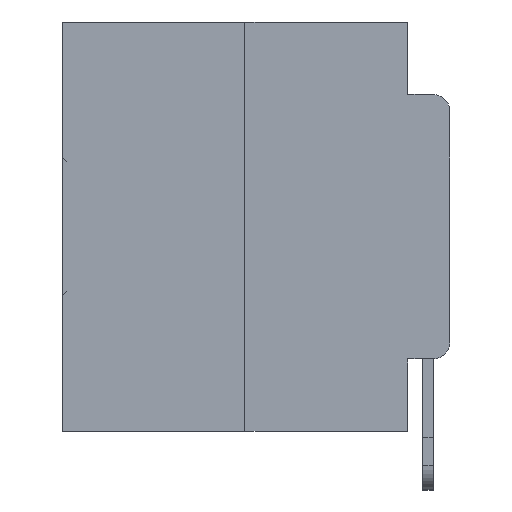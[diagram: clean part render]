
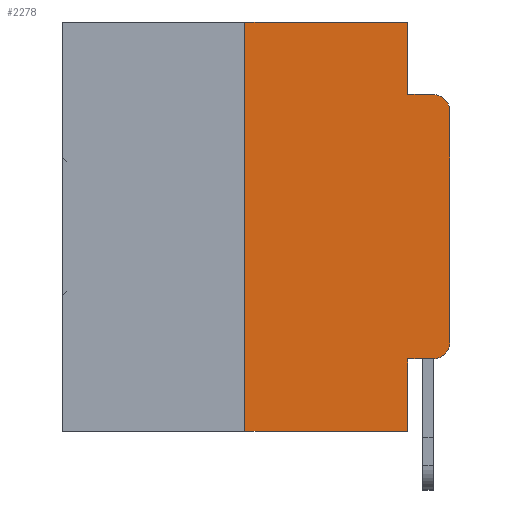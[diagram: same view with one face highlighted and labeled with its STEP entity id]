
A CAD part, left-side view. The second image highlights one B-rep face of the part: STEP entity #2278.
In plain terms, the highlighted planar face has unit normal (-1, 0, 0).
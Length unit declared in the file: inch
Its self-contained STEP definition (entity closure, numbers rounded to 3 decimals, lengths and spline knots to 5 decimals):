
#364 = EDGE_CURVE ( 'NONE', #15188, #6510, #6647, .T. ) ;
#1697 = VERTEX_POINT ( 'NONE', #27695 ) ;
#1783 = ORIENTED_EDGE ( 'NONE', *, *, #17709, .T. ) ;
#1814 = ORIENTED_EDGE ( 'NONE', *, *, #17591, .T. ) ;
#2278 = ADVANCED_FACE ( 'NONE', ( #27817 ), #11247, .F. ) ;
#2886 = EDGE_LOOP ( 'NONE', ( #29940, #19424, #7534, #15975, #30333, #12419, #1783, #5867, #1814, #16765 ) ) ;
#3053 = CIRCLE ( 'NONE', #8954, 0.02 ) ;
#3442 = VECTOR ( 'NONE', #27113, 39.37008 ) ;
#3641 = VERTEX_POINT ( 'NONE', #31999 ) ;
#3981 = EDGE_CURVE ( 'NONE', #6510, #9661, #31100, .T. ) ;
#4026 = EDGE_CURVE ( 'NONE', #1697, #14434, #3053, .T. ) ;
#4853 = DIRECTION ( 'NONE',  ( -1., 0., 0. ) ) ;
#4941 = CARTESIAN_POINT ( 'NONE',  ( 0., 0., -0.3915 ) ) ;
#5048 = CARTESIAN_POINT ( 'NONE',  ( 0., 0.473, -0.5 ) ) ;
#5867 = ORIENTED_EDGE ( 'NONE', *, *, #24782, .F. ) ;
#5984 = VECTOR ( 'NONE', #32079, 39.37008 ) ;
#6510 = VERTEX_POINT ( 'NONE', #27683 ) ;
#6591 = CARTESIAN_POINT ( 'NONE',  ( 0., 0.051, -0.5 ) ) ;
#6647 = LINE ( 'NONE', #26902, #32130 ) ;
#7245 = DIRECTION ( 'NONE',  ( 0., -1., 0. ) ) ;
#7264 = DIRECTION ( 'NONE',  ( 0., 0., -1. ) ) ;
#7534 = ORIENTED_EDGE ( 'NONE', *, *, #21222, .F. ) ;
#7689 = DIRECTION ( 'NONE',  ( 0., -1., 0. ) ) ;
#8711 = DIRECTION ( 'NONE',  ( -1., 0., 0. ) ) ;
#8758 = DIRECTION ( 'NONE',  ( 1., 0., 0. ) ) ;
#8954 = AXIS2_PLACEMENT_3D ( 'NONE', #20085, #4853, #22488 ) ;
#9661 = VERTEX_POINT ( 'NONE', #22463 ) ;
#9944 = DIRECTION ( 'NONE',  ( 0., -1., 0. ) ) ;
#10630 = AXIS2_PLACEMENT_3D ( 'NONE', #21287, #8758, #26061 ) ;
#10743 = CARTESIAN_POINT ( 'NONE',  ( 0., 0.051, -0.0885 ) ) ;
#11247 = PLANE ( 'NONE',  #10630 ) ;
#12419 = ORIENTED_EDGE ( 'NONE', *, *, #28015, .F. ) ;
#12770 = VERTEX_POINT ( 'NONE', #30619 ) ;
#12849 = VECTOR ( 'NONE', #7245, 39.37008 ) ;
#14434 = VERTEX_POINT ( 'NONE', #4941 ) ;
#15188 = VERTEX_POINT ( 'NONE', #20180 ) ;
#15628 = VECTOR ( 'NONE', #7689, 39.37008 ) ;
#15975 = ORIENTED_EDGE ( 'NONE', *, *, #3981, .F. ) ;
#16373 = LINE ( 'NONE', #5048, #15628 ) ;
#16599 = EDGE_CURVE ( 'NONE', #14434, #23954, #25861, .T. ) ;
#16765 = ORIENTED_EDGE ( 'NONE', *, *, #4026, .T. ) ;
#17411 = CARTESIAN_POINT ( 'NONE',  ( 0., 0.051, -0.4115 ) ) ;
#17591 = EDGE_CURVE ( 'NONE', #3641, #1697, #25799, .T. ) ;
#17679 = CARTESIAN_POINT ( 'NONE',  ( 0., 0., 0. ) ) ;
#17709 = EDGE_CURVE ( 'NONE', #12770, #20776, #16373, .T. ) ;
#19424 = ORIENTED_EDGE ( 'NONE', *, *, #26911, .T. ) ;
#20085 = CARTESIAN_POINT ( 'NONE',  ( 0., 0.02, -0.3915 ) ) ;
#20180 = CARTESIAN_POINT ( 'NONE',  ( 0., 0.25, 0. ) ) ;
#20213 = DIRECTION ( 'NONE',  ( 0., 0., -1. ) ) ;
#20776 = VERTEX_POINT ( 'NONE', #6591 ) ;
#21158 = CIRCLE ( 'NONE', #30148, 0.02 ) ;
#21222 = EDGE_CURVE ( 'NONE', #9661, #25954, #31265, .T. ) ;
#21287 = CARTESIAN_POINT ( 'NONE',  ( 0., 0.473, 0. ) ) ;
#21637 = VECTOR ( 'NONE', #20213, 39.37008 ) ;
#22463 = CARTESIAN_POINT ( 'NONE',  ( 0., 0.051, -0.0885 ) ) ;
#22488 = DIRECTION ( 'NONE',  ( 0., 0., -1. ) ) ;
#22758 = CARTESIAN_POINT ( 'NONE',  ( 0., 0.02, -0.0885 ) ) ;
#22789 = LINE ( 'NONE', #24657, #3442 ) ;
#23171 = VECTOR ( 'NONE', #7264, 39.37008 ) ;
#23609 = CARTESIAN_POINT ( 'NONE',  ( 0., 0.02, -0.1085 ) ) ;
#23954 = VERTEX_POINT ( 'NONE', #24697 ) ;
#24085 = VECTOR ( 'NONE', #28017, 39.37008 ) ;
#24644 = CARTESIAN_POINT ( 'NONE',  ( 0., 0.051, 0. ) ) ;
#24657 = CARTESIAN_POINT ( 'NONE',  ( 0., 0.25, 0. ) ) ;
#24697 = CARTESIAN_POINT ( 'NONE',  ( 0., 0., -0.1085 ) ) ;
#24782 = EDGE_CURVE ( 'NONE', #3641, #20776, #27980, .T. ) ;
#24881 = CARTESIAN_POINT ( 'NONE',  ( 0., 0.051, 0. ) ) ;
#25799 = LINE ( 'NONE', #17411, #12849 ) ;
#25861 = LINE ( 'NONE', #17679, #5984 ) ;
#25954 = VERTEX_POINT ( 'NONE', #22758 ) ;
#26024 = DIRECTION ( 'NONE',  ( 0., 0., -1. ) ) ;
#26061 = DIRECTION ( 'NONE',  ( 0., 0., -1. ) ) ;
#26902 = CARTESIAN_POINT ( 'NONE',  ( 0., 0.473, 0. ) ) ;
#26911 = EDGE_CURVE ( 'NONE', #23954, #25954, #21158, .T. ) ;
#27113 = DIRECTION ( 'NONE',  ( 0., 0., 1. ) ) ;
#27683 = CARTESIAN_POINT ( 'NONE',  ( 0., 0.051, 0. ) ) ;
#27695 = CARTESIAN_POINT ( 'NONE',  ( 0., 0.02, -0.4115 ) ) ;
#27817 = FACE_OUTER_BOUND ( 'NONE', #2886, .T. ) ;
#27980 = LINE ( 'NONE', #24881, #21637 ) ;
#28015 = EDGE_CURVE ( 'NONE', #12770, #15188, #22789, .T. ) ;
#28017 = DIRECTION ( 'NONE',  ( 0., -1., 0. ) ) ;
#29940 = ORIENTED_EDGE ( 'NONE', *, *, #16599, .T. ) ;
#30148 = AXIS2_PLACEMENT_3D ( 'NONE', #23609, #8711, #26024 ) ;
#30333 = ORIENTED_EDGE ( 'NONE', *, *, #364, .F. ) ;
#30619 = CARTESIAN_POINT ( 'NONE',  ( 0., 0.25, -0.5 ) ) ;
#31100 = LINE ( 'NONE', #24644, #23171 ) ;
#31265 = LINE ( 'NONE', #10743, #24085 ) ;
#31999 = CARTESIAN_POINT ( 'NONE',  ( 0., 0.051, -0.4115 ) ) ;
#32079 = DIRECTION ( 'NONE',  ( 0., 0., 1. ) ) ;
#32130 = VECTOR ( 'NONE', #9944, 39.37008 ) ;
